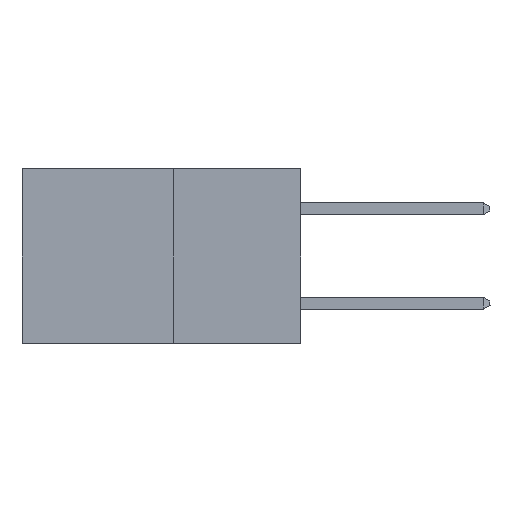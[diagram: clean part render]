
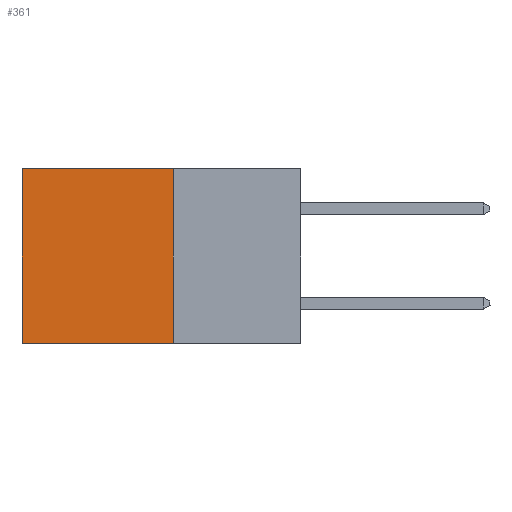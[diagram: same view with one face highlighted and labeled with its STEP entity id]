
A CAD part, left-side view. The second image highlights one B-rep face of the part: STEP entity #361.
In plain terms, the highlighted planar face has unit normal (-1, 0, 0).
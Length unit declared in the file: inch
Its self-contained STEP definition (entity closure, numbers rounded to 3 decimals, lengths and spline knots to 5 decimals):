
#361 = ADVANCED_FACE ( 'NONE', ( #15685 ), #14286, .F. ) ;
#799 = CARTESIAN_POINT ( 'NONE',  ( 0.277, 0.27, -0.37 ) ) ;
#1145 = DIRECTION ( 'NONE',  ( 0., 1., 0. ) ) ;
#1833 = DIRECTION ( 'NONE',  ( 0., 0., -1. ) ) ;
#1929 = LINE ( 'NONE', #15175, #22459 ) ;
#2364 = EDGE_LOOP ( 'NONE', ( #11522, #24191, #22058, #5432 ) ) ;
#2834 = DIRECTION ( 'NONE',  ( 0., 0., -1. ) ) ;
#3684 = CARTESIAN_POINT ( 'NONE',  ( 0.277, 0.27, 0. ) ) ;
#3859 = VERTEX_POINT ( 'NONE', #13065 ) ;
#5432 = ORIENTED_EDGE ( 'NONE', *, *, #25388, .T. ) ;
#7025 = VERTEX_POINT ( 'NONE', #3684 ) ;
#7266 = EDGE_CURVE ( 'NONE', #26438, #3859, #16887, .T. ) ;
#8477 = CARTESIAN_POINT ( 'NONE',  ( 0.277, 0.27, -0.37 ) ) ;
#9233 = LINE ( 'NONE', #20297, #14700 ) ;
#11480 = VECTOR ( 'NONE', #1145, 39.37008 ) ;
#11522 = ORIENTED_EDGE ( 'NONE', *, *, #17447, .T. ) ;
#11536 = DIRECTION ( 'NONE',  ( 0., 1., 0. ) ) ;
#12221 = VECTOR ( 'NONE', #11536, 39.37008 ) ;
#13065 = CARTESIAN_POINT ( 'NONE',  ( 0.277, 0.59, -0.37 ) ) ;
#14197 = CARTESIAN_POINT ( 'NONE',  ( 0.277, 0.59, 0. ) ) ;
#14286 = PLANE ( 'NONE',  #21342 ) ;
#14700 = VECTOR ( 'NONE', #1833, 39.37008 ) ;
#15175 = CARTESIAN_POINT ( 'NONE',  ( 0.277, 0.59, -0.37 ) ) ;
#15685 = FACE_OUTER_BOUND ( 'NONE', #2364, .T. ) ;
#15854 = VERTEX_POINT ( 'NONE', #14197 ) ;
#15882 = EDGE_CURVE ( 'NONE', #7025, #26438, #9233, .T. ) ;
#16496 = DIRECTION ( 'NONE',  ( 0., 0., -1. ) ) ;
#16887 = LINE ( 'NONE', #799, #11480 ) ;
#17447 = EDGE_CURVE ( 'NONE', #15854, #3859, #1929, .T. ) ;
#18623 = CARTESIAN_POINT ( 'NONE',  ( 0.277, 0.27, -0.37 ) ) ;
#20297 = CARTESIAN_POINT ( 'NONE',  ( 0.277, 0.27, -0.37 ) ) ;
#21342 = AXIS2_PLACEMENT_3D ( 'NONE', #8477, #25093, #16496 ) ;
#22058 = ORIENTED_EDGE ( 'NONE', *, *, #15882, .F. ) ;
#22459 = VECTOR ( 'NONE', #2834, 39.37008 ) ;
#24191 = ORIENTED_EDGE ( 'NONE', *, *, #7266, .F. ) ;
#25093 = DIRECTION ( 'NONE',  ( 1., 0., 0. ) ) ;
#25388 = EDGE_CURVE ( 'NONE', #7025, #15854, #26433, .T. ) ;
#25709 = CARTESIAN_POINT ( 'NONE',  ( 0.277, 0.27, 0. ) ) ;
#26433 = LINE ( 'NONE', #25709, #12221 ) ;
#26438 = VERTEX_POINT ( 'NONE', #18623 ) ;
